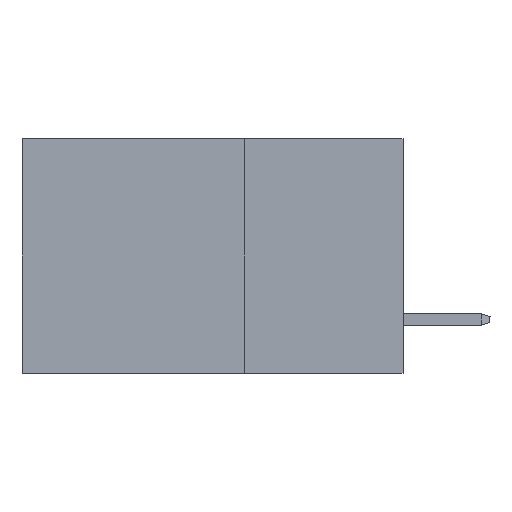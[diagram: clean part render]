
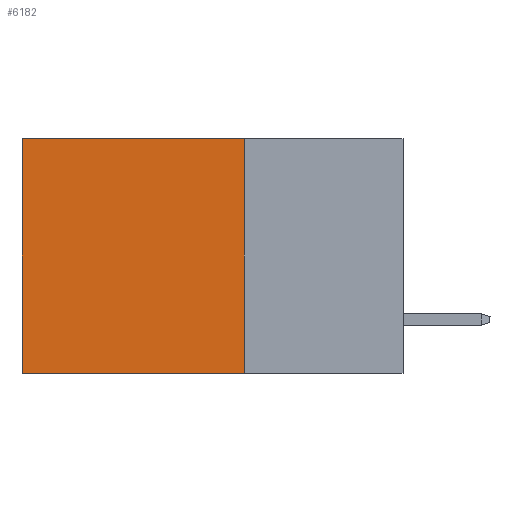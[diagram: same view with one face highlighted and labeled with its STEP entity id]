
A CAD part, left-side view. The second image highlights one B-rep face of the part: STEP entity #6182.
In plain terms, the highlighted planar face has unit normal (-1, 0, 0).
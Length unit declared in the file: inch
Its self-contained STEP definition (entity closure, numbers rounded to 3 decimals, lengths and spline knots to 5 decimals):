
#525 = EDGE_LOOP ( 'NONE', ( #47460, #28467, #21324, #15168 ) ) ;
#1756 = DIRECTION ( 'NONE',  ( 0., 0., -1. ) ) ;
#2078 = EDGE_CURVE ( 'NONE', #25738, #32780, #15994, .T. ) ;
#2822 = CARTESIAN_POINT ( 'NONE',  ( 0.2875, 0.25, 0. ) ) ;
#2878 = LINE ( 'NONE', #10643, #4455 ) ;
#4455 = VECTOR ( 'NONE', #9903, 39.37008 ) ;
#5485 = CARTESIAN_POINT ( 'NONE',  ( 0.2875, 0.6, 0. ) ) ;
#5535 = CARTESIAN_POINT ( 'NONE',  ( 0.2875, 0.25, 0. ) ) ;
#6182 = ADVANCED_FACE ( 'NONE', ( #7228 ), #33830, .F. ) ;
#7228 = FACE_OUTER_BOUND ( 'NONE', #525, .T. ) ;
#8945 = VERTEX_POINT ( 'NONE', #26831 ) ;
#9903 = DIRECTION ( 'NONE',  ( 0., 1., 0. ) ) ;
#10598 = CARTESIAN_POINT ( 'NONE',  ( 0.2875, 0.6, 0. ) ) ;
#10643 = CARTESIAN_POINT ( 'NONE',  ( 0.2875, 0.25, -0.37 ) ) ;
#15168 = ORIENTED_EDGE ( 'NONE', *, *, #23151, .T. ) ;
#15994 = LINE ( 'NONE', #5485, #26827 ) ;
#21052 = LINE ( 'NONE', #5535, #48614 ) ;
#21324 = ORIENTED_EDGE ( 'NONE', *, *, #27173, .F. ) ;
#22522 = VERTEX_POINT ( 'NONE', #2822 ) ;
#22557 = DIRECTION ( 'NONE',  ( 0., 1., 0. ) ) ;
#23005 = DIRECTION ( 'NONE',  ( 1., 0., 0. ) ) ;
#23151 = EDGE_CURVE ( 'NONE', #22522, #25738, #33613, .T. ) ;
#25738 = VERTEX_POINT ( 'NONE', #10598 ) ;
#26521 = DIRECTION ( 'NONE',  ( 0., 0., -1. ) ) ;
#26827 = VECTOR ( 'NONE', #42878, 39.37008 ) ;
#26831 = CARTESIAN_POINT ( 'NONE',  ( 0.2875, 0.25, -0.37 ) ) ;
#27173 = EDGE_CURVE ( 'NONE', #22522, #8945, #21052, .T. ) ;
#28467 = ORIENTED_EDGE ( 'NONE', *, *, #42083, .F. ) ;
#28596 = CARTESIAN_POINT ( 'NONE',  ( 0.2875, 0.6, -0.37 ) ) ;
#32780 = VERTEX_POINT ( 'NONE', #28596 ) ;
#33613 = LINE ( 'NONE', #49207, #38701 ) ;
#33830 = PLANE ( 'NONE',  #43979 ) ;
#38701 = VECTOR ( 'NONE', #22557, 39.37008 ) ;
#42083 = EDGE_CURVE ( 'NONE', #8945, #32780, #2878, .T. ) ;
#42878 = DIRECTION ( 'NONE',  ( 0., 0., -1. ) ) ;
#43979 = AXIS2_PLACEMENT_3D ( 'NONE', #45598, #23005, #26521 ) ;
#45598 = CARTESIAN_POINT ( 'NONE',  ( 0.2875, 0.25, 0. ) ) ;
#47460 = ORIENTED_EDGE ( 'NONE', *, *, #2078, .T. ) ;
#48614 = VECTOR ( 'NONE', #1756, 39.37008 ) ;
#49207 = CARTESIAN_POINT ( 'NONE',  ( 0.2875, 0.25, 0. ) ) ;
